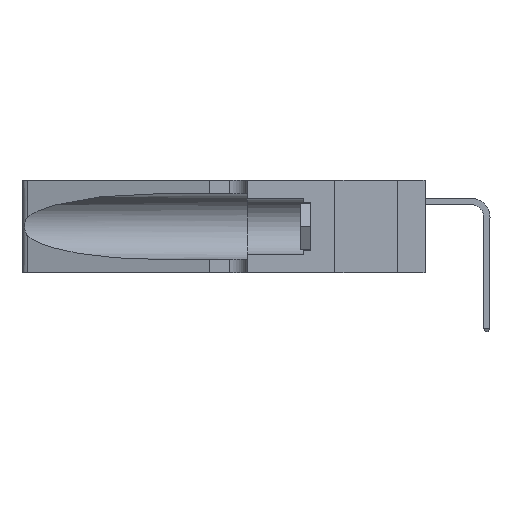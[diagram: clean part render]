
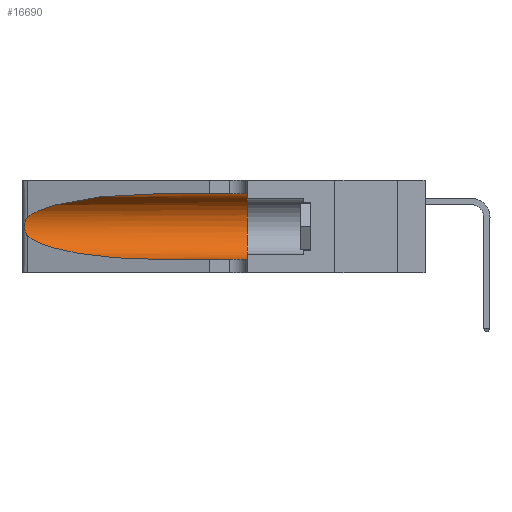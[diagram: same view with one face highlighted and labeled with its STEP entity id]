
A CAD part, left-side view. The second image highlights one B-rep face of the part: STEP entity #16690.
In plain terms, the highlighted cylindrical face has radius 3.308 mm (diameter 6.617 mm), a partial arc.
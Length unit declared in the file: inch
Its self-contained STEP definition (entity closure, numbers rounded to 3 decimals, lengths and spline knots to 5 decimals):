
#32 = LINE ( 'NONE', #18143, #24914 ) ;
#1088 = VERTEX_POINT ( 'NONE', #19311 ) ;
#1692 = CARTESIAN_POINT ( 'NONE',  ( 0.1305, 0.35, 0.31525 ) ) ;
#1798 = DIRECTION ( 'NONE',  ( 0., 0., 1. ) ) ;
#2052 = CARTESIAN_POINT ( 'NONE',  ( 0.25639, 1.23186, 0.15144 ) ) ;
#2118 =( BOUNDED_CURVE ( )  B_SPLINE_CURVE ( 3, ( #23978, #16946, #26303, #12365 ),
 .UNSPECIFIED., .F., .F. ) 
 B_SPLINE_CURVE_WITH_KNOTS ( ( 4, 4 ),
 ( 1.5708, 2.84003 ),
 .UNSPECIFIED. ) 
 CURVE ( )  GEOMETRIC_REPRESENTATION_ITEM ( )  RATIONAL_B_SPLINE_CURVE ( ( 1., 0.87, 0.87, 1. ) ) 
 REPRESENTATION_ITEM ( '' )  );
#3035 = CARTESIAN_POINT ( 'NONE',  ( 0.1305, 0.72297, 0.05475 ) ) ;
#3309 = LINE ( 'NONE', #19290, #21977 ) ;
#4107 = VERTEX_POINT ( 'NONE', #7457 ) ;
#4141 = DIRECTION ( 'NONE',  ( 0., -1., 0. ) ) ;
#4445 = CARTESIAN_POINT ( 'NONE',  ( 0.25487, 1.22718, 0.14631 ) ) ;
#4651 = ORIENTED_EDGE ( 'NONE', *, *, #15137, .T. ) ;
#5161 = CARTESIAN_POINT ( 'NONE',  ( 0.1305, 1.61858, 0.185 ) ) ;
#5299 = DIRECTION ( 'NONE',  ( 0., -1., 0. ) ) ;
#5714 = B_SPLINE_CURVE_WITH_KNOTS ( 'NONE', 3,
 ( #27603, #11284, #6681, #23004, #9022, #25354, #11392, #27698, #13747, #30017, #16080, #2052, #18441, #4445 ),
 .UNSPECIFIED., .F., .F.,
 ( 4, 2, 2, 2, 2, 2, 4 ),
 ( 0., 0.00027, 0.00053, 0.00107, 0.0016, 0.00187, 0.00214 ),
 .UNSPECIFIED. ) ;
#6515 = VERTEX_POINT ( 'NONE', #25822 ) ;
#6681 = CARTESIAN_POINT ( 'NONE',  ( 0.25639, 1.23184, 0.21858 ) ) ;
#7284 = EDGE_CURVE ( 'NONE', #6515, #24355, #10001, .T. ) ;
#7457 = CARTESIAN_POINT ( 'NONE',  ( 0.25487, 1.22718, 0.22369 ) ) ;
#9022 = CARTESIAN_POINT ( 'NONE',  ( 0.25854, 1.2359, 0.20912 ) ) ;
#9078 = FACE_OUTER_BOUND ( 'NONE', #20171, .T. ) ;
#9089 = VERTEX_POINT ( 'NONE', #29799 ) ;
#9384 = ORIENTED_EDGE ( 'NONE', *, *, #15179, .T. ) ;
#9584 = ORIENTED_EDGE ( 'NONE', *, *, #17406, .F. ) ;
#9674 = VERTEX_POINT ( 'NONE', #1692 ) ;
#10001 =( BOUNDED_CURVE ( )  B_SPLINE_CURVE ( 3, ( #12338, #14590, #17031, #3035 ),
 .UNSPECIFIED., .F., .T. ) 
 B_SPLINE_CURVE_WITH_KNOTS ( ( 4, 4 ),
 ( 3.44316, 4.71239 ),
 .UNSPECIFIED. ) 
 CURVE ( )  GEOMETRIC_REPRESENTATION_ITEM ( )  RATIONAL_B_SPLINE_CURVE ( ( 1., 0.87, 0.87, 1. ) ) 
 REPRESENTATION_ITEM ( '' )  );
#10338 = AXIS2_PLACEMENT_3D ( 'NONE', #5161, #16710, #16810 ) ;
#11284 = CARTESIAN_POINT ( 'NONE',  ( 0.25555, 1.22994, 0.2215 ) ) ;
#11392 = CARTESIAN_POINT ( 'NONE',  ( 0.26075, 1.23896, 0.19203 ) ) ;
#12338 = CARTESIAN_POINT ( 'NONE',  ( 0.25487, 1.22718, 0.14631 ) ) ;
#12365 = CARTESIAN_POINT ( 'NONE',  ( 0.25487, 1.22718, 0.22369 ) ) ;
#13747 = CARTESIAN_POINT ( 'NONE',  ( 0.26017, 1.23833, 0.17102 ) ) ;
#14590 = CARTESIAN_POINT ( 'NONE',  ( 0.2373, 1.15595, 0.08982 ) ) ;
#15137 = EDGE_CURVE ( 'NONE', #24355, #9089, #32, .T. ) ;
#15179 = EDGE_CURVE ( 'NONE', #4107, #6515, #5714, .T. ) ;
#15834 = DIRECTION ( 'NONE',  ( 0., 1., 0. ) ) ;
#16055 = EDGE_CURVE ( 'NONE', #1088, #9674, #3309, .T. ) ;
#16080 = CARTESIAN_POINT ( 'NONE',  ( 0.25789, 1.23486, 0.15765 ) ) ;
#16088 = EDGE_CURVE ( 'NONE', #1088, #4107, #2118, .T. ) ;
#16690 = ADVANCED_FACE ( 'NONE', ( #9078 ), #20783, .F. ) ;
#16710 = DIRECTION ( 'NONE',  ( 0., -1., 0. ) ) ;
#16810 = DIRECTION ( 'NONE',  ( 0., 0., -1. ) ) ;
#16946 = CARTESIAN_POINT ( 'NONE',  ( 0.18966, 0.96281, 0.31525 ) ) ;
#17031 = CARTESIAN_POINT ( 'NONE',  ( 0.18966, 0.96281, 0.05475 ) ) ;
#17072 = ORIENTED_EDGE ( 'NONE', *, *, #16055, .F. ) ;
#17406 = EDGE_CURVE ( 'NONE', #9674, #9089, #25087, .T. ) ;
#18143 = CARTESIAN_POINT ( 'NONE',  ( 0.1305, 1.61858, 0.05475 ) ) ;
#18441 = CARTESIAN_POINT ( 'NONE',  ( 0.25555, 1.22993, 0.14849 ) ) ;
#19290 = CARTESIAN_POINT ( 'NONE',  ( 0.1305, 1.61858, 0.31525 ) ) ;
#19311 = CARTESIAN_POINT ( 'NONE',  ( 0.1305, 0.72297, 0.31525 ) ) ;
#19861 = ORIENTED_EDGE ( 'NONE', *, *, #7284, .T. ) ;
#20171 = EDGE_LOOP ( 'NONE', ( #25785, #9384, #19861, #4651, #9584, #17072 ) ) ;
#20783 = CYLINDRICAL_SURFACE ( 'NONE', #10338, 0.13025 ) ;
#21977 = VECTOR ( 'NONE', #5299, 39.37008 ) ;
#23004 = CARTESIAN_POINT ( 'NONE',  ( 0.25787, 1.23484, 0.2124 ) ) ;
#23978 = CARTESIAN_POINT ( 'NONE',  ( 0.1305, 0.72297, 0.31525 ) ) ;
#24355 = VERTEX_POINT ( 'NONE', #26360 ) ;
#24914 = VECTOR ( 'NONE', #4141, 39.37008 ) ;
#25087 = CIRCLE ( 'NONE', #30054, 0.13025 ) ;
#25354 = CARTESIAN_POINT ( 'NONE',  ( 0.26018, 1.23835, 0.19895 ) ) ;
#25785 = ORIENTED_EDGE ( 'NONE', *, *, #16088, .T. ) ;
#25822 = CARTESIAN_POINT ( 'NONE',  ( 0.25487, 1.22718, 0.14631 ) ) ;
#26303 = CARTESIAN_POINT ( 'NONE',  ( 0.2373, 1.15595, 0.28018 ) ) ;
#26360 = CARTESIAN_POINT ( 'NONE',  ( 0.1305, 0.72297, 0.05475 ) ) ;
#27603 = CARTESIAN_POINT ( 'NONE',  ( 0.25487, 1.22718, 0.22369 ) ) ;
#27698 = CARTESIAN_POINT ( 'NONE',  ( 0.26075, 1.23896, 0.178 ) ) ;
#29764 = CARTESIAN_POINT ( 'NONE',  ( 0.1305, 0.35, 0.185 ) ) ;
#29799 = CARTESIAN_POINT ( 'NONE',  ( 0.1305, 0.35, 0.05475 ) ) ;
#30017 = CARTESIAN_POINT ( 'NONE',  ( 0.25856, 1.23593, 0.16098 ) ) ;
#30054 = AXIS2_PLACEMENT_3D ( 'NONE', #29764, #15834, #1798 ) ;
